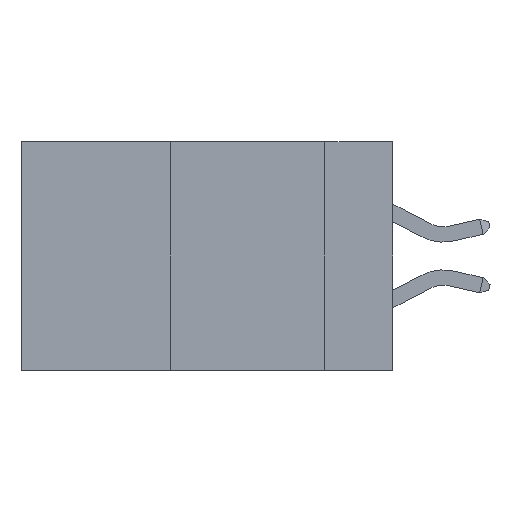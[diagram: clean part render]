
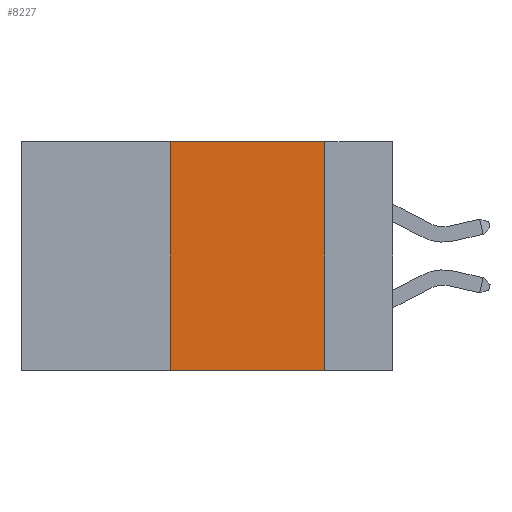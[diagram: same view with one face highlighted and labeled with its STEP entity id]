
A CAD part, left-side view. The second image highlights one B-rep face of the part: STEP entity #8227.
In plain terms, the highlighted planar face has unit normal (-1, 0, 0).
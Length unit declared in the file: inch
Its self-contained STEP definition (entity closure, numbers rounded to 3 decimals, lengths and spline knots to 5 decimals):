
#737 = VERTEX_POINT ( 'NONE', #15249 ) ;
#1112 = AXIS2_PLACEMENT_3D ( 'NONE', #1454, #14377, #13076 ) ;
#1216 = DIRECTION ( 'NONE',  ( 0., 0., 1. ) ) ;
#1441 = CARTESIAN_POINT ( 'NONE',  ( 0., 0.11, 0. ) ) ;
#1454 = CARTESIAN_POINT ( 'NONE',  ( 0., 0.6, 0. ) ) ;
#1726 = LINE ( 'NONE', #6692, #11735 ) ;
#2445 = EDGE_LOOP ( 'NONE', ( #16904, #8285, #16966, #18192 ) ) ;
#3085 = VECTOR ( 'NONE', #6338, 39.37008 ) ;
#3326 = FACE_OUTER_BOUND ( 'NONE', #2445, .T. ) ;
#4198 = PLANE ( 'NONE',  #1112 ) ;
#4928 = CARTESIAN_POINT ( 'NONE',  ( 0., 0.36, 0. ) ) ;
#6338 = DIRECTION ( 'NONE',  ( 0., -1., 0. ) ) ;
#6692 = CARTESIAN_POINT ( 'NONE',  ( 0., 0.11, 0. ) ) ;
#6796 = VECTOR ( 'NONE', #17834, 39.37008 ) ;
#7520 = EDGE_CURVE ( 'NONE', #11291, #13078, #1726, .T. ) ;
#8227 = ADVANCED_FACE ( 'NONE', ( #3326 ), #4198, .F. ) ;
#8285 = ORIENTED_EDGE ( 'NONE', *, *, #13101, .F. ) ;
#8445 = CARTESIAN_POINT ( 'NONE',  ( 0., 0.36, 0. ) ) ;
#8492 = LINE ( 'NONE', #16346, #3085 ) ;
#9439 = EDGE_CURVE ( 'NONE', #737, #14128, #15391, .T. ) ;
#10530 = VECTOR ( 'NONE', #1216, 39.37008 ) ;
#11291 = VERTEX_POINT ( 'NONE', #1441 ) ;
#11735 = VECTOR ( 'NONE', #18410, 39.37008 ) ;
#12038 = LINE ( 'NONE', #13673, #6796 ) ;
#13076 = DIRECTION ( 'NONE',  ( 0., 0., -1. ) ) ;
#13078 = VERTEX_POINT ( 'NONE', #17901 ) ;
#13101 = EDGE_CURVE ( 'NONE', #14128, #11291, #12038, .T. ) ;
#13673 = CARTESIAN_POINT ( 'NONE',  ( 0., 0.6, 0. ) ) ;
#14128 = VERTEX_POINT ( 'NONE', #4928 ) ;
#14377 = DIRECTION ( 'NONE',  ( 1., 0., 0. ) ) ;
#15249 = CARTESIAN_POINT ( 'NONE',  ( 0., 0.36, -0.37 ) ) ;
#15274 = EDGE_CURVE ( 'NONE', #737, #13078, #8492, .T. ) ;
#15391 = LINE ( 'NONE', #8445, #10530 ) ;
#16346 = CARTESIAN_POINT ( 'NONE',  ( 0., 0.6, -0.37 ) ) ;
#16904 = ORIENTED_EDGE ( 'NONE', *, *, #7520, .F. ) ;
#16966 = ORIENTED_EDGE ( 'NONE', *, *, #9439, .F. ) ;
#17834 = DIRECTION ( 'NONE',  ( 0., -1., 0. ) ) ;
#17901 = CARTESIAN_POINT ( 'NONE',  ( 0., 0.11, -0.37 ) ) ;
#18192 = ORIENTED_EDGE ( 'NONE', *, *, #15274, .T. ) ;
#18410 = DIRECTION ( 'NONE',  ( 0., 0., -1. ) ) ;
